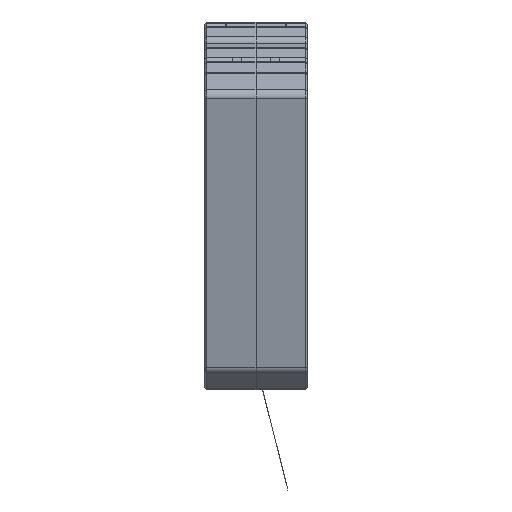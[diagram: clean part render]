
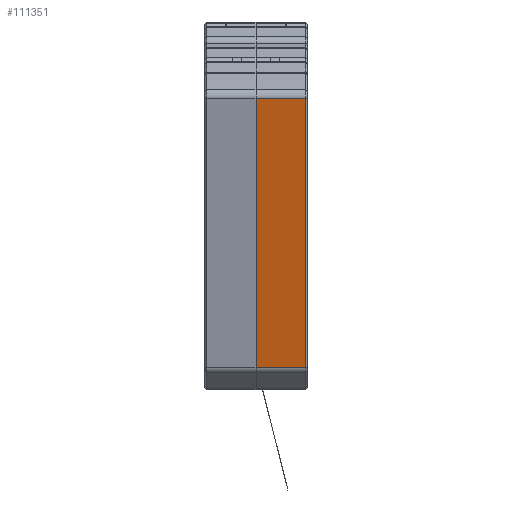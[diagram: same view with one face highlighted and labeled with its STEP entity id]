
A CAD part, front view. The second image highlights one B-rep face of the part: STEP entity #111351.
In plain terms, the highlighted planar face has unit normal (0, -0.97, -0.241).
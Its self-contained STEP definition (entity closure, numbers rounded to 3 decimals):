
#2081 = EDGE_CURVE ( 'NONE', #7218, #17065, #8932, .T. ) ;
#3772 = ORIENTED_EDGE ( 'NONE', *, *, #58487, .T. ) ;
#4403 = LINE ( 'NONE', #14040, #83293 ) ;
#5837 = EDGE_LOOP ( 'NONE', ( #3772, #5915, #91506, #69964 ) ) ;
#5915 = ORIENTED_EDGE ( 'NONE', *, *, #2081, .T. ) ;
#6546 = CARTESIAN_POINT ( 'NONE',  ( 79.551, -105.317, -26.203 ) ) ;
#7218 = VERTEX_POINT ( 'NONE', #7302 ) ;
#7302 = CARTESIAN_POINT ( 'NONE',  ( 12.252, -101.021, -43.469 ) ) ;
#8932 = LINE ( 'NONE', #61747, #57439 ) ;
#14040 = CARTESIAN_POINT ( 'NONE',  ( 0., -105.317, -26.203 ) ) ;
#17065 = VERTEX_POINT ( 'NONE', #26460 ) ;
#17545 = FACE_OUTER_BOUND ( 'NONE', #5837, .T. ) ;
#26460 = CARTESIAN_POINT ( 'NONE',  ( 12.252, -117.611, 23.208 ) ) ;
#29956 = DIRECTION ( 'NONE',  ( 1., 0., 0. ) ) ;
#35728 = DIRECTION ( 'NONE',  ( -1., 0., 0. ) ) ;
#40164 = DIRECTION ( 'NONE',  ( 0., -0.97, -0.241 ) ) ;
#40302 = CARTESIAN_POINT ( 'NONE',  ( 35.962, -117.611, 23.208 ) ) ;
#57439 = VECTOR ( 'NONE', #94058, 1000. ) ;
#58097 = CARTESIAN_POINT ( 'NONE',  ( 79.551, -101.021, -43.469 ) ) ;
#58487 = EDGE_CURVE ( 'NONE', #88778, #7218, #132919, .T. ) ;
#60730 = PLANE ( 'NONE',  #114266 ) ;
#61747 = CARTESIAN_POINT ( 'NONE',  ( 12.252, -105.317, -26.203 ) ) ;
#68438 = CARTESIAN_POINT ( 'NONE',  ( 0., -101.021, -43.469 ) ) ;
#69964 = ORIENTED_EDGE ( 'NONE', *, *, #99770, .F. ) ;
#70687 = EDGE_CURVE ( 'NONE', #17065, #120835, #102761, .T. ) ;
#80749 = CARTESIAN_POINT ( 'NONE',  ( 0., -117.611, 23.208 ) ) ;
#83293 = VECTOR ( 'NONE', #84802, 1000. ) ;
#84466 = VECTOR ( 'NONE', #29956, 1000. ) ;
#84802 = DIRECTION ( 'NONE',  ( 0., -0.241, 0.97 ) ) ;
#88778 = VERTEX_POINT ( 'NONE', #68438 ) ;
#91506 = ORIENTED_EDGE ( 'NONE', *, *, #70687, .T. ) ;
#94058 = DIRECTION ( 'NONE',  ( 0., -0.241, 0.97 ) ) ;
#94697 = VECTOR ( 'NONE', #35728, 1000. ) ;
#99770 = EDGE_CURVE ( 'NONE', #88778, #120835, #4403, .T. ) ;
#101946 = DIRECTION ( 'NONE',  ( 0., 0.241, -0.97 ) ) ;
#102761 = LINE ( 'NONE', #40302, #94697 ) ;
#111351 = ADVANCED_FACE ( 'NONE', ( #17545 ), #60730, .T. ) ;
#114266 = AXIS2_PLACEMENT_3D ( 'NONE', #6546, #40164, #101946 ) ;
#120835 = VERTEX_POINT ( 'NONE', #80749 ) ;
#132919 = LINE ( 'NONE', #58097, #84466 ) ;
